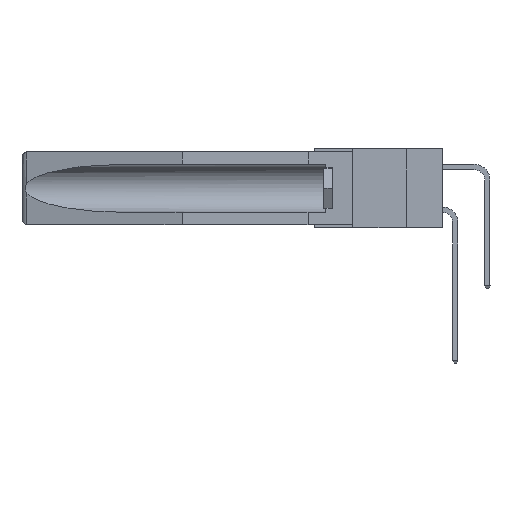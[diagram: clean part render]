
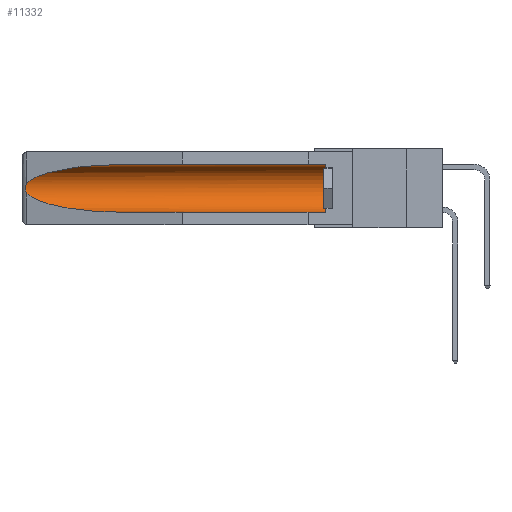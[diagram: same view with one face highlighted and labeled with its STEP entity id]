
A CAD part, left-side view. The second image highlights one B-rep face of the part: STEP entity #11332.
In plain terms, the highlighted cylindrical face has radius 2.857 mm (diameter 5.715 mm), a partial arc.
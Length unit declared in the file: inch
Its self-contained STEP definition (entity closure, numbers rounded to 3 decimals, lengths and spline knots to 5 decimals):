
#331 = DIRECTION ( 'NONE',  ( 0., 1., 0. ) ) ;
#692 = LINE ( 'NONE', #23005, #10432 ) ;
#907 = CARTESIAN_POINT ( 'NONE',  ( 0.155, 1.07973, -0.059 ) ) ;
#1306 = B_SPLINE_CURVE_WITH_KNOTS ( 'NONE', 3,
 ( #6525, #13194, #17665, #21912, #4356, #3052, #20807, #16494, #22915, #18297 ),
 .UNSPECIFIED., .F., .F.,
 ( 4, 2, 2, 2, 4 ),
 ( 0., 0.00029, 0.00058, 0.00087, 0.00117 ),
 .UNSPECIFIED. ) ;
#1671 =( BOUNDED_CURVE ( )  B_SPLINE_CURVE ( 3, ( #18014, #24379, #26599, #20126 ),
 .UNSPECIFIED., .F., .F. ) 
 B_SPLINE_CURVE_WITH_KNOTS ( ( 4, 4 ),
 ( 4.71239, 6.08839 ),
 .UNSPECIFIED. ) 
 CURVE ( )  GEOMETRIC_REPRESENTATION_ITEM ( )  RATIONAL_B_SPLINE_CURVE ( ( 1., 0.848, 0.848, 1. ) ) 
 REPRESENTATION_ITEM ( '' )  );
#2173 = ORIENTED_EDGE ( 'NONE', *, *, #11676, .T. ) ;
#2276 = CARTESIAN_POINT ( 'NONE',  ( 0.155, -0.30754, -0.059 ) ) ;
#2403 = EDGE_CURVE ( 'NONE', #24392, #18190, #692, .T. ) ;
#3052 = CARTESIAN_POINT ( 'NONE',  ( 0.2675, 1.53308, -0.17534 ) ) ;
#3442 = VERTEX_POINT ( 'NONE', #907 ) ;
#4323 = VERTEX_POINT ( 'NONE', #14738 ) ;
#4356 = CARTESIAN_POINT ( 'NONE',  ( 0.2675, 1.53308, -0.16763 ) ) ;
#5673 = DIRECTION ( 'NONE',  ( 0., 1., 0. ) ) ;
#5868 = EDGE_CURVE ( 'NONE', #24392, #10018, #25190, .T. ) ;
#6386 = EDGE_CURVE ( 'NONE', #4323, #15695, #1306, .T. ) ;
#6525 = CARTESIAN_POINT ( 'NONE',  ( 0.26537, 1.52718, -0.14972 ) ) ;
#7558 = DIRECTION ( 'NONE',  ( 0., -1., 0. ) ) ;
#8100 = CARTESIAN_POINT ( 'NONE',  ( 0.155, -0.30754, -0.1715 ) ) ;
#10018 = VERTEX_POINT ( 'NONE', #16846 ) ;
#10432 = VECTOR ( 'NONE', #12169, 39.37008 ) ;
#11176 = FACE_OUTER_BOUND ( 'NONE', #23190, .T. ) ;
#11332 = ADVANCED_FACE ( 'NONE', ( #11176 ), #17005, .F. ) ;
#11676 = EDGE_CURVE ( 'NONE', #10018, #3442, #15810, .T. ) ;
#11692 = ORIENTED_EDGE ( 'NONE', *, *, #2403, .F. ) ;
#12023 = DIRECTION ( 'NONE',  ( 0., 0., 1. ) ) ;
#12169 = DIRECTION ( 'NONE',  ( 0., 1., 0. ) ) ;
#12365 = VECTOR ( 'NONE', #331, 39.37008 ) ;
#12755 = CARTESIAN_POINT ( 'NONE',  ( 0.25451, 1.48313, -0.24835 ) ) ;
#12832 = CARTESIAN_POINT ( 'NONE',  ( 0.155, 1.07973, -0.284 ) ) ;
#13194 = CARTESIAN_POINT ( 'NONE',  ( 0.26597, 1.52961, -0.15275 ) ) ;
#13999 = CARTESIAN_POINT ( 'NONE',  ( 0.155, 0.126, -0.284 ) ) ;
#14227 = CARTESIAN_POINT ( 'NONE',  ( 0.155, 0.126, -0.1715 ) ) ;
#14675 = CARTESIAN_POINT ( 'NONE',  ( 0.26537, 1.52718, -0.19328 ) ) ;
#14738 = CARTESIAN_POINT ( 'NONE',  ( 0.26537, 1.52718, -0.14972 ) ) ;
#15501 = AXIS2_PLACEMENT_3D ( 'NONE', #8100, #5673, #17134 ) ;
#15695 = VERTEX_POINT ( 'NONE', #14675 ) ;
#15810 = LINE ( 'NONE', #2276, #12365 ) ;
#16065 = CARTESIAN_POINT ( 'NONE',  ( 0.155, 1.07973, -0.284 ) ) ;
#16175 = AXIS2_PLACEMENT_3D ( 'NONE', #14227, #7558, #12023 ) ;
#16494 = CARTESIAN_POINT ( 'NONE',  ( 0.26655, 1.53094, -0.18657 ) ) ;
#16846 = CARTESIAN_POINT ( 'NONE',  ( 0.155, 0.126, -0.059 ) ) ;
#17005 = CYLINDRICAL_SURFACE ( 'NONE', #15501, 0.1125 ) ;
#17134 = DIRECTION ( 'NONE',  ( 0., 0., 1. ) ) ;
#17665 = CARTESIAN_POINT ( 'NONE',  ( 0.26654, 1.53092, -0.15636 ) ) ;
#18014 = CARTESIAN_POINT ( 'NONE',  ( 0.155, 1.07973, -0.059 ) ) ;
#18190 = VERTEX_POINT ( 'NONE', #16065 ) ;
#18297 = CARTESIAN_POINT ( 'NONE',  ( 0.26537, 1.52718, -0.19328 ) ) ;
#18591 = EDGE_CURVE ( 'NONE', #3442, #4323, #1671, .T. ) ;
#19052 = ORIENTED_EDGE ( 'NONE', *, *, #6386, .T. ) ;
#19704 =( BOUNDED_CURVE ( )  B_SPLINE_CURVE ( 3, ( #23580, #12755, #26255, #12832 ),
 .UNSPECIFIED., .F., .F. ) 
 B_SPLINE_CURVE_WITH_KNOTS ( ( 4, 4 ),
 ( 0.1948, 1.5708 ),
 .UNSPECIFIED. ) 
 CURVE ( )  GEOMETRIC_REPRESENTATION_ITEM ( )  RATIONAL_B_SPLINE_CURVE ( ( 1., 0.848, 0.848, 1. ) ) 
 REPRESENTATION_ITEM ( '' )  );
#19756 = ORIENTED_EDGE ( 'NONE', *, *, #27132, .T. ) ;
#20090 = ORIENTED_EDGE ( 'NONE', *, *, #5868, .T. ) ;
#20126 = CARTESIAN_POINT ( 'NONE',  ( 0.26537, 1.52718, -0.14972 ) ) ;
#20807 = CARTESIAN_POINT ( 'NONE',  ( 0.2673, 1.53269, -0.17917 ) ) ;
#21912 = CARTESIAN_POINT ( 'NONE',  ( 0.2673, 1.5327, -0.16383 ) ) ;
#22608 = ORIENTED_EDGE ( 'NONE', *, *, #18591, .T. ) ;
#22915 = CARTESIAN_POINT ( 'NONE',  ( 0.26597, 1.5296, -0.19026 ) ) ;
#23005 = CARTESIAN_POINT ( 'NONE',  ( 0.155, -0.30754, -0.284 ) ) ;
#23190 = EDGE_LOOP ( 'NONE', ( #22608, #19052, #19756, #11692, #20090, #2173 ) ) ;
#23580 = CARTESIAN_POINT ( 'NONE',  ( 0.26537, 1.52718, -0.19328 ) ) ;
#24379 = CARTESIAN_POINT ( 'NONE',  ( 0.21114, 1.30732, -0.059 ) ) ;
#24392 = VERTEX_POINT ( 'NONE', #13999 ) ;
#25190 = CIRCLE ( 'NONE', #16175, 0.1125 ) ;
#26255 = CARTESIAN_POINT ( 'NONE',  ( 0.21114, 1.30732, -0.284 ) ) ;
#26599 = CARTESIAN_POINT ( 'NONE',  ( 0.25451, 1.48313, -0.09465 ) ) ;
#27132 = EDGE_CURVE ( 'NONE', #15695, #18190, #19704, .T. ) ;
